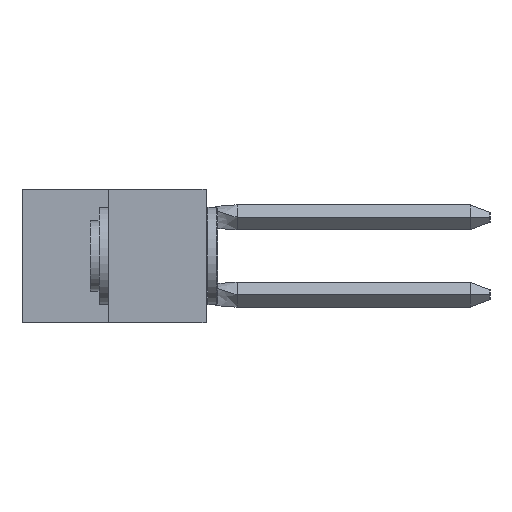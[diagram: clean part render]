
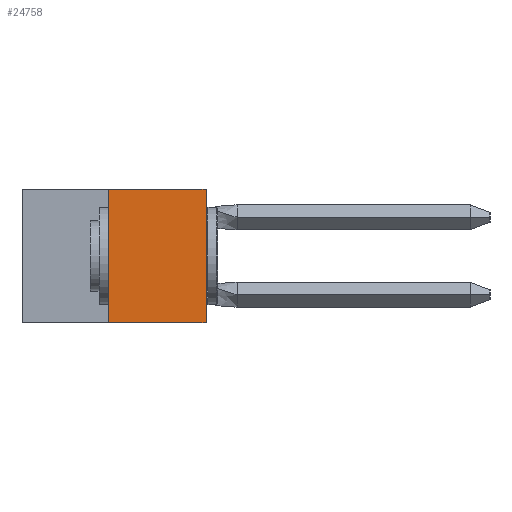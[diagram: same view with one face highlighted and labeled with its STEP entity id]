
A CAD part, left-side view. The second image highlights one B-rep face of the part: STEP entity #24758.
In plain terms, the highlighted planar face has unit normal (-1, 0, 0).
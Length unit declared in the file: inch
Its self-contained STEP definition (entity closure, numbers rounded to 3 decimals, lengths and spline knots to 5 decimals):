
#6 = VECTOR ( 'NONE', #2431, 39.37008 ) ;
#2213 = ORIENTED_EDGE ( 'NONE', *, *, #2749, .F. ) ;
#2431 = DIRECTION ( 'NONE',  ( 0., -1., 0. ) ) ;
#2749 = EDGE_CURVE ( 'NONE', #4374, #15596, #3575, .T. ) ;
#3575 = LINE ( 'NONE', #26653, #36725 ) ;
#4374 = VERTEX_POINT ( 'NONE', #8720 ) ;
#5154 = ORIENTED_EDGE ( 'NONE', *, *, #23956, .T. ) ;
#5698 = PLANE ( 'NONE',  #17444 ) ;
#6840 = ORIENTED_EDGE ( 'NONE', *, *, #36877, .F. ) ;
#8720 = CARTESIAN_POINT ( 'NONE',  ( 0., 0.25, -0.343 ) ) ;
#12319 = VERTEX_POINT ( 'NONE', #13452 ) ;
#13132 = ORIENTED_EDGE ( 'NONE', *, *, #36862, .T. ) ;
#13452 = CARTESIAN_POINT ( 'NONE',  ( 0., 0., 0. ) ) ;
#14321 = CARTESIAN_POINT ( 'NONE',  ( 0., 0.473, -0.343 ) ) ;
#15596 = VERTEX_POINT ( 'NONE', #22377 ) ;
#17444 = AXIS2_PLACEMENT_3D ( 'NONE', #20934, #27676, #29353 ) ;
#19356 = LINE ( 'NONE', #37609, #34301 ) ;
#20280 = CARTESIAN_POINT ( 'NONE',  ( 0., 0.473, 0. ) ) ;
#20413 = DIRECTION ( 'NONE',  ( 0., -1., 0. ) ) ;
#20550 = DIRECTION ( 'NONE',  ( 0., 0., 1. ) ) ;
#20934 = CARTESIAN_POINT ( 'NONE',  ( 0., 0.473, 0. ) ) ;
#20999 = LINE ( 'NONE', #14321, #36903 ) ;
#21595 = FACE_OUTER_BOUND ( 'NONE', #26409, .T. ) ;
#22377 = CARTESIAN_POINT ( 'NONE',  ( 0., 0.25, 0. ) ) ;
#23956 = EDGE_CURVE ( 'NONE', #27740, #12319, #19356, .T. ) ;
#24758 = ADVANCED_FACE ( 'NONE', ( #21595 ), #5698, .F. ) ;
#25686 = DIRECTION ( 'NONE',  ( 0., 0., 1. ) ) ;
#26409 = EDGE_LOOP ( 'NONE', ( #6840, #2213, #13132, #5154 ) ) ;
#26603 = LINE ( 'NONE', #20280, #6 ) ;
#26653 = CARTESIAN_POINT ( 'NONE',  ( 0., 0.25, 0. ) ) ;
#27676 = DIRECTION ( 'NONE',  ( 1., 0., 0. ) ) ;
#27740 = VERTEX_POINT ( 'NONE', #36743 ) ;
#29353 = DIRECTION ( 'NONE',  ( 0., 0., -1. ) ) ;
#34301 = VECTOR ( 'NONE', #25686, 39.37008 ) ;
#36725 = VECTOR ( 'NONE', #20550, 39.37008 ) ;
#36743 = CARTESIAN_POINT ( 'NONE',  ( 0., 0., -0.343 ) ) ;
#36862 = EDGE_CURVE ( 'NONE', #4374, #27740, #20999, .T. ) ;
#36877 = EDGE_CURVE ( 'NONE', #15596, #12319, #26603, .T. ) ;
#36903 = VECTOR ( 'NONE', #20413, 39.37008 ) ;
#37609 = CARTESIAN_POINT ( 'NONE',  ( 0., 0., 0. ) ) ;
